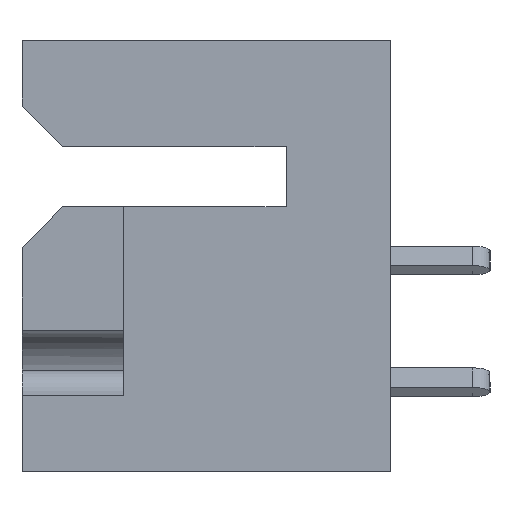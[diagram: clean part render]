
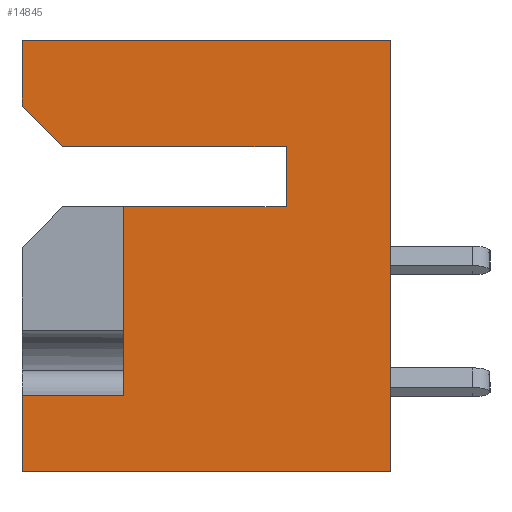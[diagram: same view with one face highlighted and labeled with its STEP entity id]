
A CAD part, left-side view. The second image highlights one B-rep face of the part: STEP entity #14845.
In plain terms, the highlighted planar face has unit normal (-1, 0, 0).
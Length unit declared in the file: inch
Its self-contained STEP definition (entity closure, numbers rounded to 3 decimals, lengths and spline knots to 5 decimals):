
#43 = CARTESIAN_POINT ( 'NONE',  ( 0., 0.328, -0.437 ) ) ;
#570 = CARTESIAN_POINT ( 'NONE',  ( 0., 0.453, -0.531 ) ) ;
#1112 = EDGE_CURVE ( 'NONE', #25576, #6929, #21612, .T. ) ;
#1218 = VECTOR ( 'NONE', #24685, 39.37008 ) ;
#1385 = CARTESIAN_POINT ( 'NONE',  ( 0., 0.453, -0.531 ) ) ;
#1715 = VERTEX_POINT ( 'NONE', #24509 ) ;
#1879 = LINE ( 'NONE', #21391, #20489 ) ;
#2019 = CARTESIAN_POINT ( 'NONE',  ( 0., 0., -0.531 ) ) ;
#2446 = DIRECTION ( 'NONE',  ( 0., 1., 0. ) ) ;
#2591 = EDGE_CURVE ( 'NONE', #16435, #4225, #12172, .T. ) ;
#3082 = EDGE_CURVE ( 'NONE', #1715, #26461, #19491, .T. ) ;
#3106 = DIRECTION ( 'NONE',  ( 0., 1., 0. ) ) ;
#3339 = LINE ( 'NONE', #18763, #14552 ) ;
#4225 = VERTEX_POINT ( 'NONE', #5795 ) ;
#4275 = DIRECTION ( 'NONE',  ( 0., 0., 1. ) ) ;
#5419 = CARTESIAN_POINT ( 'NONE',  ( 0., 0., 0. ) ) ;
#5677 = CARTESIAN_POINT ( 'NONE',  ( 0., 0.128, -0.131 ) ) ;
#5795 = CARTESIAN_POINT ( 'NONE',  ( 0., 0.403, -0.131 ) ) ;
#6184 = ORIENTED_EDGE ( 'NONE', *, *, #15566, .T. ) ;
#6546 = DIRECTION ( 'NONE',  ( 0., 0., 1. ) ) ;
#6929 = VERTEX_POINT ( 'NONE', #22673 ) ;
#7414 = VECTOR ( 'NONE', #2446, 39.37008 ) ;
#7875 = FACE_OUTER_BOUND ( 'NONE', #22395, .T. ) ;
#8245 = VECTOR ( 'NONE', #26333, 39.37008 ) ;
#8251 = EDGE_CURVE ( 'NONE', #6929, #29430, #12860, .T. ) ;
#8290 = VECTOR ( 'NONE', #3106, 39.37008 ) ;
#8597 = VECTOR ( 'NONE', #25719, 39.37008 ) ;
#8714 = ORIENTED_EDGE ( 'NONE', *, *, #21111, .T. ) ;
#8801 = ORIENTED_EDGE ( 'NONE', *, *, #19789, .F. ) ;
#9979 = AXIS2_PLACEMENT_3D ( 'NONE', #20188, #27921, #22504 ) ;
#11279 = CARTESIAN_POINT ( 'NONE',  ( 0., 0.453, -0.081 ) ) ;
#11606 = VERTEX_POINT ( 'NONE', #28942 ) ;
#11607 = DIRECTION ( 'NONE',  ( 0., -0.707, -0.707 ) ) ;
#12172 = LINE ( 'NONE', #17807, #8290 ) ;
#12860 = LINE ( 'NONE', #20694, #8597 ) ;
#13272 = EDGE_CURVE ( 'NONE', #11606, #26461, #21186, .T. ) ;
#13442 = VECTOR ( 'NONE', #4275, 39.37008 ) ;
#13634 = LINE ( 'NONE', #43, #7414 ) ;
#13804 = ORIENTED_EDGE ( 'NONE', *, *, #3082, .T. ) ;
#14152 = CARTESIAN_POINT ( 'NONE',  ( 0., 0., 0. ) ) ;
#14179 = VECTOR ( 'NONE', #31536, 39.37008 ) ;
#14478 = LINE ( 'NONE', #1385, #8245 ) ;
#14552 = VECTOR ( 'NONE', #11607, 39.37008 ) ;
#14654 = ORIENTED_EDGE ( 'NONE', *, *, #8251, .F. ) ;
#14845 = ADVANCED_FACE ( 'NONE', ( #7875 ), #22920, .F. ) ;
#14951 = LINE ( 'NONE', #14152, #14179 ) ;
#15566 = EDGE_CURVE ( 'NONE', #31598, #21950, #14478, .T. ) ;
#16417 = CARTESIAN_POINT ( 'NONE',  ( 0., 0.128, -0.131 ) ) ;
#16435 = VERTEX_POINT ( 'NONE', #5677 ) ;
#16902 = ORIENTED_EDGE ( 'NONE', *, *, #17804, .T. ) ;
#17804 = EDGE_CURVE ( 'NONE', #11606, #24604, #13634, .T. ) ;
#17807 = CARTESIAN_POINT ( 'NONE',  ( 0., 0.128, -0.131 ) ) ;
#18450 = ORIENTED_EDGE ( 'NONE', *, *, #2591, .F. ) ;
#18763 = CARTESIAN_POINT ( 'NONE',  ( 0., 0.403, -0.131 ) ) ;
#19491 = LINE ( 'NONE', #25390, #28078 ) ;
#19789 = EDGE_CURVE ( 'NONE', #31598, #24604, #1879, .T. ) ;
#20188 = CARTESIAN_POINT ( 'NONE',  ( 0., 0.453, 0. ) ) ;
#20312 = DIRECTION ( 'NONE',  ( 0., 0., 1. ) ) ;
#20489 = VECTOR ( 'NONE', #6546, 39.37008 ) ;
#20694 = CARTESIAN_POINT ( 'NONE',  ( 0., 0.453, 0. ) ) ;
#21111 = EDGE_CURVE ( 'NONE', #21950, #29430, #14951, .T. ) ;
#21186 = LINE ( 'NONE', #30002, #22354 ) ;
#21368 = LINE ( 'NONE', #16417, #1218 ) ;
#21391 = CARTESIAN_POINT ( 'NONE',  ( 0., 0.453, 0. ) ) ;
#21612 = LINE ( 'NONE', #28913, #13442 ) ;
#21950 = VERTEX_POINT ( 'NONE', #2019 ) ;
#22354 = VECTOR ( 'NONE', #20312, 39.37008 ) ;
#22395 = EDGE_LOOP ( 'NONE', ( #16902, #8801, #6184, #8714, #14654, #24210, #22856, #18450, #23933, #13804, #25029 ) ) ;
#22504 = DIRECTION ( 'NONE',  ( 0., 0., -1. ) ) ;
#22673 = CARTESIAN_POINT ( 'NONE',  ( 0., 0.453, 0. ) ) ;
#22856 = ORIENTED_EDGE ( 'NONE', *, *, #25729, .T. ) ;
#22920 = PLANE ( 'NONE',  #9979 ) ;
#23087 = DIRECTION ( 'NONE',  ( 0., 1., 0. ) ) ;
#23933 = ORIENTED_EDGE ( 'NONE', *, *, #28672, .F. ) ;
#24210 = ORIENTED_EDGE ( 'NONE', *, *, #1112, .F. ) ;
#24509 = CARTESIAN_POINT ( 'NONE',  ( 0., 0.128, -0.205 ) ) ;
#24604 = VERTEX_POINT ( 'NONE', #29842 ) ;
#24685 = DIRECTION ( 'NONE',  ( 0., 0., 1. ) ) ;
#25029 = ORIENTED_EDGE ( 'NONE', *, *, #13272, .F. ) ;
#25390 = CARTESIAN_POINT ( 'NONE',  ( 0., 0.128, -0.205 ) ) ;
#25576 = VERTEX_POINT ( 'NONE', #11279 ) ;
#25719 = DIRECTION ( 'NONE',  ( 0., -1., 0. ) ) ;
#25729 = EDGE_CURVE ( 'NONE', #25576, #4225, #3339, .T. ) ;
#26333 = DIRECTION ( 'NONE',  ( 0., -1., 0. ) ) ;
#26461 = VERTEX_POINT ( 'NONE', #29065 ) ;
#27921 = DIRECTION ( 'NONE',  ( 1., 0., 0. ) ) ;
#28078 = VECTOR ( 'NONE', #23087, 39.37008 ) ;
#28672 = EDGE_CURVE ( 'NONE', #1715, #16435, #21368, .T. ) ;
#28913 = CARTESIAN_POINT ( 'NONE',  ( 0., 0.453, 0. ) ) ;
#28942 = CARTESIAN_POINT ( 'NONE',  ( 0., 0.328, -0.437 ) ) ;
#29065 = CARTESIAN_POINT ( 'NONE',  ( 0., 0.328, -0.205 ) ) ;
#29430 = VERTEX_POINT ( 'NONE', #5419 ) ;
#29842 = CARTESIAN_POINT ( 'NONE',  ( 0., 0.453, -0.437 ) ) ;
#30002 = CARTESIAN_POINT ( 'NONE',  ( 0., 0.328, -0.205 ) ) ;
#31536 = DIRECTION ( 'NONE',  ( 0., 0., 1. ) ) ;
#31598 = VERTEX_POINT ( 'NONE', #570 ) ;
